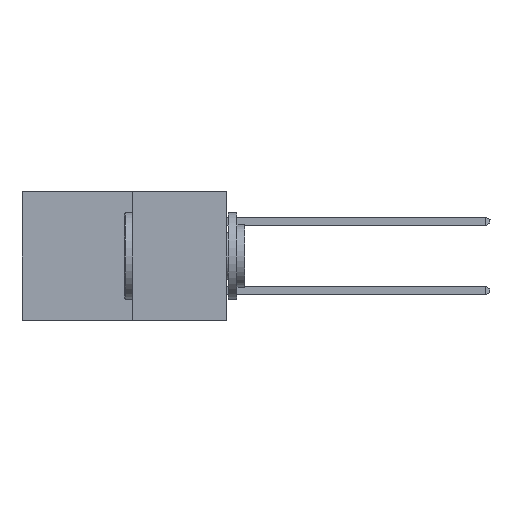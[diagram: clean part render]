
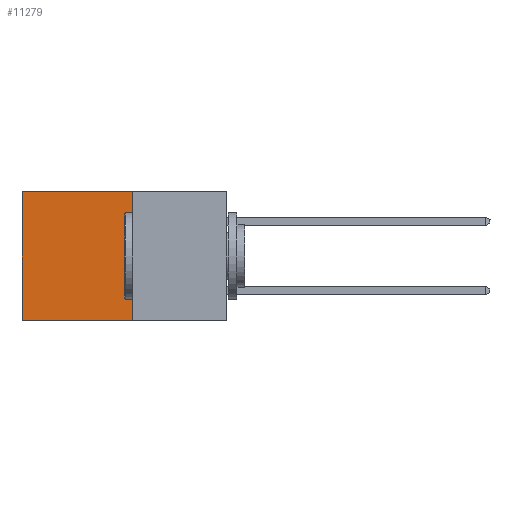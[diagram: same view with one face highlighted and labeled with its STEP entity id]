
A CAD part, left-side view. The second image highlights one B-rep face of the part: STEP entity #11279.
In plain terms, the highlighted planar face has unit normal (-1, 0, 0).
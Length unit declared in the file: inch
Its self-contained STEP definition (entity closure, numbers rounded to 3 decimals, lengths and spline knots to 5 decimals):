
#16 = CARTESIAN_POINT ( 'NONE',  ( 0.277, 0.27, -0.37 ) ) ;
#383 = VERTEX_POINT ( 'NONE', #8757 ) ;
#626 = PLANE ( 'NONE',  #15700 ) ;
#638 = EDGE_CURVE ( 'NONE', #7685, #13962, #3197, .T. ) ;
#1088 = CARTESIAN_POINT ( 'NONE',  ( 0.277, 0.59, 0. ) ) ;
#1258 = ORIENTED_EDGE ( 'NONE', *, *, #8802, .T. ) ;
#1918 = ORIENTED_EDGE ( 'NONE', *, *, #14566, .T. ) ;
#2274 = CARTESIAN_POINT ( 'NONE',  ( 0.277, 0.59, -0.37 ) ) ;
#2642 = EDGE_CURVE ( 'NONE', #13962, #383, #3761, .T. ) ;
#2957 = VECTOR ( 'NONE', #14001, 39.37008 ) ;
#3197 = LINE ( 'NONE', #16, #6168 ) ;
#3325 = DIRECTION ( 'NONE',  ( 0., 0., -1. ) ) ;
#3381 = VECTOR ( 'NONE', #6097, 39.37008 ) ;
#3761 = LINE ( 'NONE', #10725, #3381 ) ;
#4572 = DIRECTION ( 'NONE',  ( 1., 0., 0. ) ) ;
#5497 = CARTESIAN_POINT ( 'NONE',  ( 0.277, 0.27, -0.37 ) ) ;
#6097 = DIRECTION ( 'NONE',  ( 0., 1., 0. ) ) ;
#6168 = VECTOR ( 'NONE', #3325, 39.37008 ) ;
#7163 = CARTESIAN_POINT ( 'NONE',  ( 0.277, 0.27, -0.37 ) ) ;
#7685 = VERTEX_POINT ( 'NONE', #15616 ) ;
#8757 = CARTESIAN_POINT ( 'NONE',  ( 0.277, 0.59, -0.37 ) ) ;
#8802 = EDGE_CURVE ( 'NONE', #9588, #383, #16647, .T. ) ;
#9414 = DIRECTION ( 'NONE',  ( 0., 1., 0. ) ) ;
#9427 = EDGE_LOOP ( 'NONE', ( #1258, #12160, #16655, #1918 ) ) ;
#9588 = VERTEX_POINT ( 'NONE', #1088 ) ;
#10725 = CARTESIAN_POINT ( 'NONE',  ( 0.277, 0.27, -0.37 ) ) ;
#11279 = ADVANCED_FACE ( 'NONE', ( #11920 ), #626, .F. ) ;
#11920 = FACE_OUTER_BOUND ( 'NONE', #9427, .T. ) ;
#12160 = ORIENTED_EDGE ( 'NONE', *, *, #2642, .F. ) ;
#13733 = DIRECTION ( 'NONE',  ( 0., 0., -1. ) ) ;
#13962 = VERTEX_POINT ( 'NONE', #5497 ) ;
#14001 = DIRECTION ( 'NONE',  ( 0., 0., -1. ) ) ;
#14549 = VECTOR ( 'NONE', #9414, 39.37008 ) ;
#14566 = EDGE_CURVE ( 'NONE', #7685, #9588, #14932, .T. ) ;
#14932 = LINE ( 'NONE', #15765, #14549 ) ;
#15616 = CARTESIAN_POINT ( 'NONE',  ( 0.277, 0.27, 0. ) ) ;
#15700 = AXIS2_PLACEMENT_3D ( 'NONE', #7163, #4572, #13733 ) ;
#15765 = CARTESIAN_POINT ( 'NONE',  ( 0.277, 0.27, 0. ) ) ;
#16647 = LINE ( 'NONE', #2274, #2957 ) ;
#16655 = ORIENTED_EDGE ( 'NONE', *, *, #638, .F. ) ;
